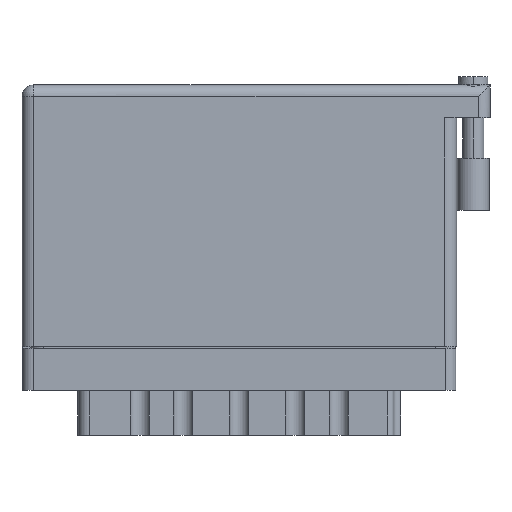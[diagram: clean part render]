
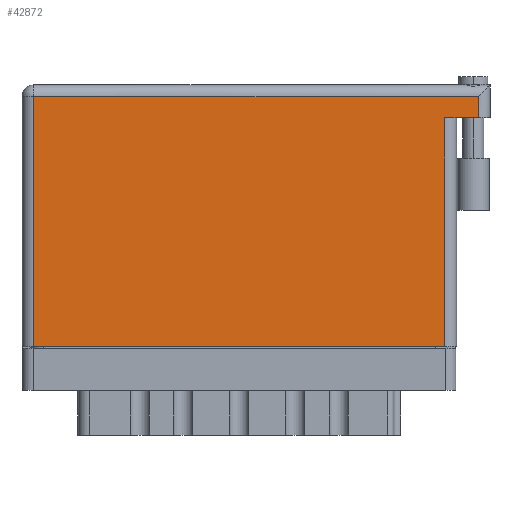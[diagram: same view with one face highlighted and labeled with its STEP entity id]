
A CAD part, front view. The second image highlights one B-rep face of the part: STEP entity #42872.
In plain terms, the highlighted face is planar.
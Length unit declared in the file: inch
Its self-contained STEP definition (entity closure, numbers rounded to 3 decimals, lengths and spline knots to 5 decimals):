
#235 = AXIS2_PLACEMENT_3D ( 'NONE', #31170, #6095, #51677 ) ;
#444 = DIRECTION ( 'NONE',  ( -1., 0., 0. ) ) ;
#2469 = CARTESIAN_POINT ( 'NONE',  ( 2.73, 1.496, 0. ) ) ;
#6095 = DIRECTION ( 'NONE',  ( 0., 0., -1. ) ) ;
#6625 = PLANE ( 'NONE',  #235 ) ;
#6885 = FACE_OUTER_BOUND ( 'NONE', #26064, .T. ) ;
#7432 = VECTOR ( 'NONE', #35965, 39.37008 ) ;
#7695 = VERTEX_POINT ( 'NONE', #13670 ) ;
#7980 = ORIENTED_EDGE ( 'NONE', *, *, #47881, .T. ) ;
#8646 = VERTEX_POINT ( 'NONE', #2469 ) ;
#9644 = CARTESIAN_POINT ( 'NONE',  ( 0.07, 0., 0. ) ) ;
#11854 = DIRECTION ( 'NONE',  ( 0., -1., 0. ) ) ;
#12615 = CARTESIAN_POINT ( 'NONE',  ( 2.53, 1.369, 0. ) ) ;
#13670 = CARTESIAN_POINT ( 'NONE',  ( 0.07, 1.496, 0. ) ) ;
#15112 = VECTOR ( 'NONE', #11854, 39.37008 ) ;
#15836 = VECTOR ( 'NONE', #51387, 39.37008 ) ;
#17218 = VERTEX_POINT ( 'NONE', #33518 ) ;
#17385 = EDGE_CURVE ( 'NONE', #8646, #7695, #26496, .T. ) ;
#18125 = DIRECTION ( 'NONE',  ( -1., 0., 0. ) ) ;
#18147 = VERTEX_POINT ( 'NONE', #9644 ) ;
#19814 = ORIENTED_EDGE ( 'NONE', *, *, #17385, .T. ) ;
#20068 = EDGE_CURVE ( 'NONE', #18147, #48958, #40020, .T. ) ;
#22818 = EDGE_CURVE ( 'NONE', #7695, #18147, #32356, .T. ) ;
#23037 = CARTESIAN_POINT ( 'NONE',  ( 2.73, 1.566, 0. ) ) ;
#24758 = DIRECTION ( 'NONE',  ( 0., 1., 0. ) ) ;
#25134 = ORIENTED_EDGE ( 'NONE', *, *, #20068, .T. ) ;
#26064 = EDGE_LOOP ( 'NONE', ( #25134, #48161, #50106, #7980, #19814, #42754 ) ) ;
#26496 = LINE ( 'NONE', #34837, #32852 ) ;
#26582 = CARTESIAN_POINT ( 'NONE',  ( 0., 0., 0. ) ) ;
#28220 = CARTESIAN_POINT ( 'NONE',  ( 2.8, 1.369, 0. ) ) ;
#29830 = EDGE_CURVE ( 'NONE', #17218, #33553, #32287, .T. ) ;
#31170 = CARTESIAN_POINT ( 'NONE',  ( 0., 1.566, 0. ) ) ;
#32199 = LINE ( 'NONE', #23037, #7432 ) ;
#32287 = LINE ( 'NONE', #28220, #37244 ) ;
#32356 = LINE ( 'NONE', #48793, #15112 ) ;
#32852 = VECTOR ( 'NONE', #18125, 39.37008 ) ;
#33518 = CARTESIAN_POINT ( 'NONE',  ( 2.73, 1.369, 0. ) ) ;
#33553 = VERTEX_POINT ( 'NONE', #35864 ) ;
#34837 = CARTESIAN_POINT ( 'NONE',  ( 0., 1.496, 0. ) ) ;
#35864 = CARTESIAN_POINT ( 'NONE',  ( 2.53, 1.369, 0. ) ) ;
#35965 = DIRECTION ( 'NONE',  ( 0., 1., 0. ) ) ;
#36865 = LINE ( 'NONE', #12615, #51938 ) ;
#37244 = VECTOR ( 'NONE', #444, 39.37008 ) ;
#40020 = LINE ( 'NONE', #26582, #15836 ) ;
#42645 = EDGE_CURVE ( 'NONE', #48958, #33553, #36865, .T. ) ;
#42754 = ORIENTED_EDGE ( 'NONE', *, *, #22818, .T. ) ;
#42872 = ADVANCED_FACE ( 'NONE', ( #6885 ), #6625, .F. ) ;
#45054 = CARTESIAN_POINT ( 'NONE',  ( 2.53, 0., 0. ) ) ;
#47881 = EDGE_CURVE ( 'NONE', #17218, #8646, #32199, .T. ) ;
#48161 = ORIENTED_EDGE ( 'NONE', *, *, #42645, .T. ) ;
#48793 = CARTESIAN_POINT ( 'NONE',  ( 0.07, 0., 0. ) ) ;
#48958 = VERTEX_POINT ( 'NONE', #45054 ) ;
#50106 = ORIENTED_EDGE ( 'NONE', *, *, #29830, .F. ) ;
#51387 = DIRECTION ( 'NONE',  ( 1., 0., 0. ) ) ;
#51677 = DIRECTION ( 'NONE',  ( -1., 0., 0. ) ) ;
#51938 = VECTOR ( 'NONE', #24758, 39.37008 ) ;
